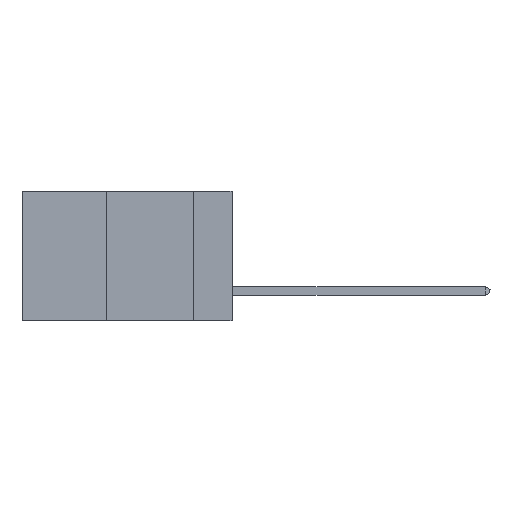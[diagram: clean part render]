
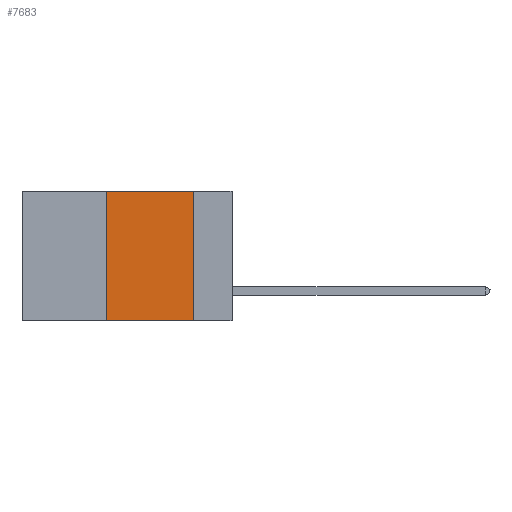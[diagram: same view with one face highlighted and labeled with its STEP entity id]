
A CAD part, left-side view. The second image highlights one B-rep face of the part: STEP entity #7683.
In plain terms, the highlighted planar face has unit normal (-1, 0, 0).
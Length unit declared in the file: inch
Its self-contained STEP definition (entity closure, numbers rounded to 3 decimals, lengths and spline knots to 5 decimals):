
#101 = DIRECTION ( 'NONE',  ( 0., 0., -1. ) ) ;
#174 = VECTOR ( 'NONE', #11423, 39.37008 ) ;
#2446 = PLANE ( 'NONE',  #3730 ) ;
#3263 = LINE ( 'NONE', #5512, #174 ) ;
#3434 = VERTEX_POINT ( 'NONE', #13753 ) ;
#3582 = DIRECTION ( 'NONE',  ( 0., 0., 1. ) ) ;
#3730 = AXIS2_PLACEMENT_3D ( 'NONE', #7142, #14022, #101 ) ;
#4286 = CARTESIAN_POINT ( 'NONE',  ( 0., 0.36, 0. ) ) ;
#4429 = VECTOR ( 'NONE', #7388, 39.37008 ) ;
#4585 = ORIENTED_EDGE ( 'NONE', *, *, #8765, .F. ) ;
#4807 = CARTESIAN_POINT ( 'NONE',  ( 0., 0.6, -0.37 ) ) ;
#5133 = CARTESIAN_POINT ( 'NONE',  ( 0., 0.11, -0.37 ) ) ;
#5223 = LINE ( 'NONE', #4807, #13995 ) ;
#5512 = CARTESIAN_POINT ( 'NONE',  ( 0., 0.6, 0. ) ) ;
#5669 = EDGE_LOOP ( 'NONE', ( #11724, #4585, #7726, #10801 ) ) ;
#6291 = EDGE_CURVE ( 'NONE', #3434, #13928, #9863, .T. ) ;
#7142 = CARTESIAN_POINT ( 'NONE',  ( 0., 0.6, 0. ) ) ;
#7388 = DIRECTION ( 'NONE',  ( 0., 0., -1. ) ) ;
#7662 = VERTEX_POINT ( 'NONE', #4286 ) ;
#7683 = ADVANCED_FACE ( 'NONE', ( #9462 ), #2446, .F. ) ;
#7726 = ORIENTED_EDGE ( 'NONE', *, *, #8476, .F. ) ;
#8110 = CARTESIAN_POINT ( 'NONE',  ( 0., 0.11, 0. ) ) ;
#8171 = LINE ( 'NONE', #9558, #8358 ) ;
#8358 = VECTOR ( 'NONE', #3582, 39.37008 ) ;
#8476 = EDGE_CURVE ( 'NONE', #9828, #7662, #8171, .T. ) ;
#8765 = EDGE_CURVE ( 'NONE', #7662, #3434, #3263, .T. ) ;
#9462 = FACE_OUTER_BOUND ( 'NONE', #5669, .T. ) ;
#9558 = CARTESIAN_POINT ( 'NONE',  ( 0., 0.36, 0. ) ) ;
#9828 = VERTEX_POINT ( 'NONE', #12916 ) ;
#9863 = LINE ( 'NONE', #8110, #4429 ) ;
#10651 = EDGE_CURVE ( 'NONE', #9828, #13928, #5223, .T. ) ;
#10801 = ORIENTED_EDGE ( 'NONE', *, *, #10651, .T. ) ;
#11423 = DIRECTION ( 'NONE',  ( 0., -1., 0. ) ) ;
#11724 = ORIENTED_EDGE ( 'NONE', *, *, #6291, .F. ) ;
#11828 = DIRECTION ( 'NONE',  ( 0., -1., 0. ) ) ;
#12916 = CARTESIAN_POINT ( 'NONE',  ( 0., 0.36, -0.37 ) ) ;
#13753 = CARTESIAN_POINT ( 'NONE',  ( 0., 0.11, 0. ) ) ;
#13928 = VERTEX_POINT ( 'NONE', #5133 ) ;
#13995 = VECTOR ( 'NONE', #11828, 39.37008 ) ;
#14022 = DIRECTION ( 'NONE',  ( 1., 0., 0. ) ) ;
